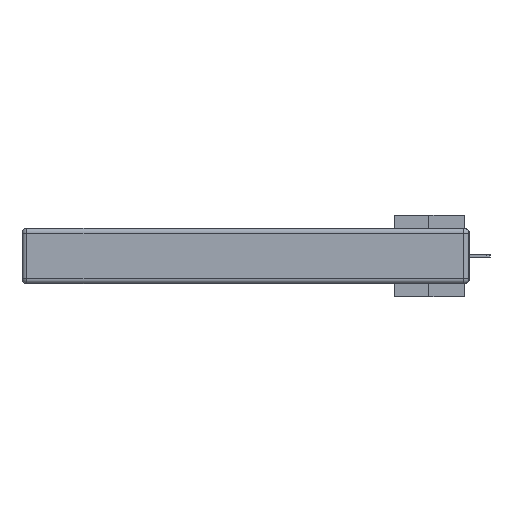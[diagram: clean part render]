
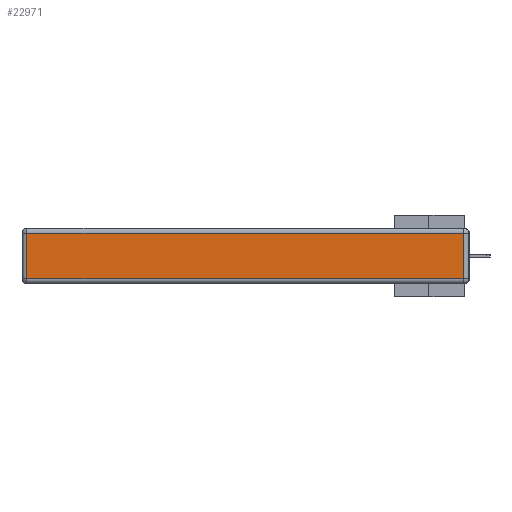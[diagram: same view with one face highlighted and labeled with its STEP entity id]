
A CAD part, left-side view. The second image highlights one B-rep face of the part: STEP entity #22971.
In plain terms, the highlighted planar face has unit normal (-1, 0, 0).
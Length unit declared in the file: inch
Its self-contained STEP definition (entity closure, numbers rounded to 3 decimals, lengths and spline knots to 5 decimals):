
#1708 = VECTOR ( 'NONE', #31056, 39.37008 ) ;
#2837 = VERTEX_POINT ( 'NONE', #19473 ) ;
#3349 = VECTOR ( 'NONE', #10779, 39.37008 ) ;
#3671 = CARTESIAN_POINT ( 'NONE',  ( 0., 2.75, -0.03 ) ) ;
#4416 = ORIENTED_EDGE ( 'NONE', *, *, #8093, .T. ) ;
#5143 = FACE_OUTER_BOUND ( 'NONE', #7921, .T. ) ;
#7921 = EDGE_LOOP ( 'NONE', ( #33538, #11538, #25545, #4416 ) ) ;
#8017 = CARTESIAN_POINT ( 'NONE',  ( 0., 0.03, -0.343 ) ) ;
#8093 = EDGE_CURVE ( 'NONE', #33489, #2837, #10160, .T. ) ;
#10016 = DIRECTION ( 'NONE',  ( 0., 0., -1. ) ) ;
#10160 = LINE ( 'NONE', #20982, #15741 ) ;
#10669 = DIRECTION ( 'NONE',  ( 0., 0., 1. ) ) ;
#10779 = DIRECTION ( 'NONE',  ( 0., 0., 1. ) ) ;
#11031 = AXIS2_PLACEMENT_3D ( 'NONE', #35060, #27030, #10669 ) ;
#11175 = CARTESIAN_POINT ( 'NONE',  ( 0., 2.72, -0.03 ) ) ;
#11538 = ORIENTED_EDGE ( 'NONE', *, *, #19844, .T. ) ;
#14102 = VERTEX_POINT ( 'NONE', #32385 ) ;
#15739 = DIRECTION ( 'NONE',  ( 0., -1., 0. ) ) ;
#15741 = VECTOR ( 'NONE', #10016, 39.37008 ) ;
#19473 = CARTESIAN_POINT ( 'NONE',  ( 0., 2.72, -0.313 ) ) ;
#19844 = EDGE_CURVE ( 'NONE', #14102, #29112, #25263, .T. ) ;
#20982 = CARTESIAN_POINT ( 'NONE',  ( 0., 2.72, -0.343 ) ) ;
#21253 = CARTESIAN_POINT ( 'NONE',  ( 0., 0.03, -0.03 ) ) ;
#21628 = PLANE ( 'NONE',  #11031 ) ;
#22971 = ADVANCED_FACE ( 'NONE', ( #5143 ), #21628, .T. ) ;
#25263 = LINE ( 'NONE', #8017, #3349 ) ;
#25545 = ORIENTED_EDGE ( 'NONE', *, *, #27085, .T. ) ;
#27030 = DIRECTION ( 'NONE',  ( -1., 0., 0. ) ) ;
#27085 = EDGE_CURVE ( 'NONE', #29112, #33489, #31719, .T. ) ;
#29112 = VERTEX_POINT ( 'NONE', #21253 ) ;
#29336 = CARTESIAN_POINT ( 'NONE',  ( 0., 0., -0.313 ) ) ;
#31056 = DIRECTION ( 'NONE',  ( 0., 1., 0. ) ) ;
#31194 = EDGE_CURVE ( 'NONE', #2837, #14102, #33558, .T. ) ;
#31719 = LINE ( 'NONE', #3671, #1708 ) ;
#32385 = CARTESIAN_POINT ( 'NONE',  ( 0., 0.03, -0.313 ) ) ;
#32700 = VECTOR ( 'NONE', #15739, 39.37008 ) ;
#33489 = VERTEX_POINT ( 'NONE', #11175 ) ;
#33538 = ORIENTED_EDGE ( 'NONE', *, *, #31194, .T. ) ;
#33558 = LINE ( 'NONE', #29336, #32700 ) ;
#35060 = CARTESIAN_POINT ( 'NONE',  ( 0., 0., -0.343 ) ) ;
